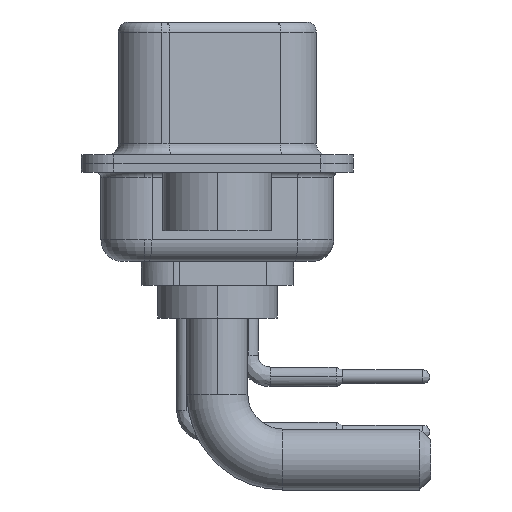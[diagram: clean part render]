
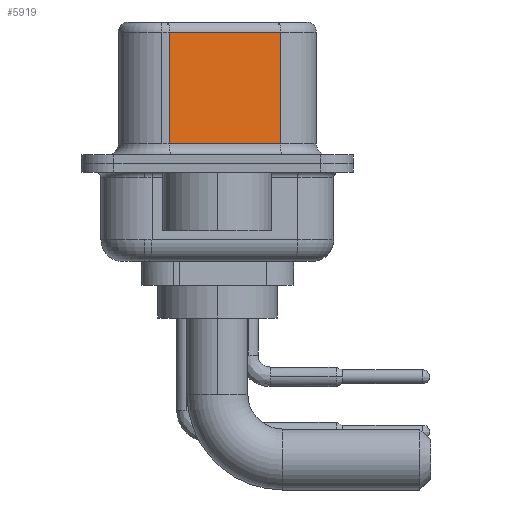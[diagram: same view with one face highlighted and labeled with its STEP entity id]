
A CAD part, left-side view. The second image highlights one B-rep face of the part: STEP entity #5919.
In plain terms, the highlighted planar face has unit normal (-0.985, -0.174, 0).
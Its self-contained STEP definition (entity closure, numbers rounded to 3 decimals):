
#128 = DIRECTION ( 'NONE',  ( 0., 0., -1. ) ) ;
#338 = ORIENTED_EDGE ( 'NONE', *, *, #14886, .T. ) ;
#523 = EDGE_LOOP ( 'NONE', ( #7170, #15054, #6952, #338 ) ) ;
#636 = DIRECTION ( 'NONE',  ( 0.174, -0.985, 0. ) ) ;
#764 = VECTOR ( 'NONE', #128, 1000. ) ;
#1202 = DIRECTION ( 'NONE',  ( -0.174, 0.985, 0. ) ) ;
#1658 = VERTEX_POINT ( 'NONE', #4598 ) ;
#2250 = VECTOR ( 'NONE', #636, 1000. ) ;
#2604 = EDGE_CURVE ( 'NONE', #8963, #22081, #5971, .T. ) ;
#4426 = LINE ( 'NONE', #21946, #23297 ) ;
#4598 = CARTESIAN_POINT ( 'NONE',  ( 3.68, 2.203, 6.02 ) ) ;
#5919 = ADVANCED_FACE ( 'NONE', ( #11192 ), #13263, .F. ) ;
#5971 = LINE ( 'NONE', #17905, #764 ) ;
#6952 = ORIENTED_EDGE ( 'NONE', *, *, #7193, .T. ) ;
#7170 = ORIENTED_EDGE ( 'NONE', *, *, #2604, .F. ) ;
#7193 = EDGE_CURVE ( 'NONE', #1658, #9396, #9290, .T. ) ;
#8772 = CARTESIAN_POINT ( 'NONE',  ( 3.68, 2.203, 6.52 ) ) ;
#8963 = VERTEX_POINT ( 'NONE', #14704 ) ;
#9290 = LINE ( 'NONE', #8772, #11175 ) ;
#9396 = VERTEX_POINT ( 'NONE', #24688 ) ;
#10830 = CARTESIAN_POINT ( 'NONE',  ( 4.58, -2.897, 0.9 ) ) ;
#10979 = EDGE_CURVE ( 'NONE', #8963, #1658, #4426, .T. ) ;
#11175 = VECTOR ( 'NONE', #16942, 1000. ) ;
#11192 = FACE_OUTER_BOUND ( 'NONE', #523, .T. ) ;
#13129 = CARTESIAN_POINT ( 'NONE',  ( 4.58, -2.897, 6.52 ) ) ;
#13263 = PLANE ( 'NONE',  #14271 ) ;
#14271 = AXIS2_PLACEMENT_3D ( 'NONE', #13129, #25212, #1202 ) ;
#14704 = CARTESIAN_POINT ( 'NONE',  ( 4.58, -2.897, 6.02 ) ) ;
#14886 = EDGE_CURVE ( 'NONE', #9396, #22081, #18411, .T. ) ;
#15054 = ORIENTED_EDGE ( 'NONE', *, *, #10979, .T. ) ;
#16942 = DIRECTION ( 'NONE',  ( 0., 0., -1. ) ) ;
#17905 = CARTESIAN_POINT ( 'NONE',  ( 4.58, -2.897, 6.52 ) ) ;
#18055 = DIRECTION ( 'NONE',  ( -0.174, 0.985, 0. ) ) ;
#18411 = LINE ( 'NONE', #22442, #2250 ) ;
#21946 = CARTESIAN_POINT ( 'NONE',  ( 4.58, -2.897, 6.02 ) ) ;
#22081 = VERTEX_POINT ( 'NONE', #10830 ) ;
#22442 = CARTESIAN_POINT ( 'NONE',  ( 4.58, -2.897, 0.9 ) ) ;
#23297 = VECTOR ( 'NONE', #18055, 1000. ) ;
#24688 = CARTESIAN_POINT ( 'NONE',  ( 3.68, 2.203, 0.9 ) ) ;
#25212 = DIRECTION ( 'NONE',  ( 0.985, 0.174, 0. ) ) ;
